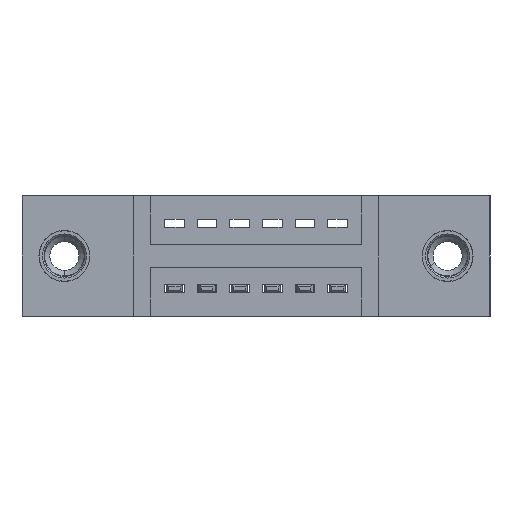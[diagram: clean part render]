
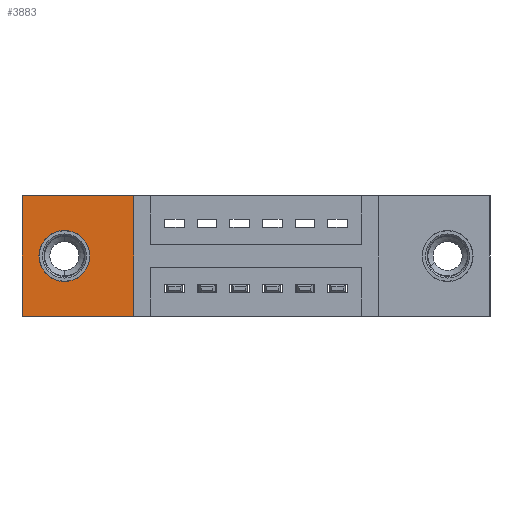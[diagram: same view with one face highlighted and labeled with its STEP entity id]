
A CAD part, front view. The second image highlights one B-rep face of the part: STEP entity #3883.
In plain terms, the highlighted planar face has unit normal (0, -1, 0).
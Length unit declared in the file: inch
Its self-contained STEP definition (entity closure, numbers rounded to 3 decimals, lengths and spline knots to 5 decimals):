
#91 = LINE ( 'NONE', #8628, #228 ) ;
#122 = DIRECTION ( 'NONE',  ( 0., -1., 0. ) ) ;
#217 = DIRECTION ( 'NONE',  ( 0., 0., -1. ) ) ;
#228 = VECTOR ( 'NONE', #3759, 39.37008 ) ;
#829 = ORIENTED_EDGE ( 'NONE', *, *, #8064, .T. ) ;
#845 = DIRECTION ( 'NONE',  ( 0., 0., -1. ) ) ;
#876 = EDGE_CURVE ( 'NONE', #2872, #4630, #8509, .T. ) ;
#2139 = ORIENTED_EDGE ( 'NONE', *, *, #2926, .T. ) ;
#2263 = FACE_BOUND ( 'NONE', #3488, .T. ) ;
#2465 = AXIS2_PLACEMENT_3D ( 'NONE', #4232, #8338, #217 ) ;
#2575 = PLANE ( 'NONE',  #2465 ) ;
#2872 = VERTEX_POINT ( 'NONE', #9754 ) ;
#2926 = EDGE_CURVE ( 'NONE', #3399, #8544, #91, .T. ) ;
#3018 = CARTESIAN_POINT ( 'NONE',  ( 0.13, 0.17, -0.185 ) ) ;
#3065 = EDGE_CURVE ( 'NONE', #5907, #3399, #10058, .T. ) ;
#3149 = ORIENTED_EDGE ( 'NONE', *, *, #876, .F. ) ;
#3399 = VERTEX_POINT ( 'NONE', #9287 ) ;
#3439 = DIRECTION ( 'NONE',  ( -1., 0., 0. ) ) ;
#3488 = EDGE_LOOP ( 'NONE', ( #5017, #3149 ) ) ;
#3630 = DIRECTION ( 'NONE',  ( 1., 0., 0. ) ) ;
#3645 = CIRCLE ( 'NONE', #3818, 0.078 ) ;
#3669 = EDGE_LOOP ( 'NONE', ( #5337, #8537, #2139, #829 ) ) ;
#3759 = DIRECTION ( 'NONE',  ( 0., 0., 1. ) ) ;
#3801 = CARTESIAN_POINT ( 'NONE',  ( 0., 0.17, 0. ) ) ;
#3818 = AXIS2_PLACEMENT_3D ( 'NONE', #3018, #7141, #4140 ) ;
#3883 = ADVANCED_FACE ( 'NONE', ( #2263, #5244 ), #2575, .T. ) ;
#3909 = DIRECTION ( 'NONE',  ( 0., 0., -1. ) ) ;
#4140 = DIRECTION ( 'NONE',  ( 0., 0., -1. ) ) ;
#4232 = CARTESIAN_POINT ( 'NONE',  ( 0., 0.17, -0.37 ) ) ;
#4376 = AXIS2_PLACEMENT_3D ( 'NONE', #5072, #122, #845 ) ;
#4400 = CARTESIAN_POINT ( 'NONE',  ( 0., 0.17, -0.37 ) ) ;
#4551 = CARTESIAN_POINT ( 'NONE',  ( 0.13, 0.17, -0.107 ) ) ;
#4630 = VERTEX_POINT ( 'NONE', #4551 ) ;
#4685 = LINE ( 'NONE', #5545, #5567 ) ;
#5017 = ORIENTED_EDGE ( 'NONE', *, *, #8403, .F. ) ;
#5072 = CARTESIAN_POINT ( 'NONE',  ( 0.13, 0.17, -0.185 ) ) ;
#5175 = LINE ( 'NONE', #8282, #7061 ) ;
#5244 = FACE_OUTER_BOUND ( 'NONE', #3669, .T. ) ;
#5337 = ORIENTED_EDGE ( 'NONE', *, *, #5396, .T. ) ;
#5396 = EDGE_CURVE ( 'NONE', #7038, #5907, #4685, .T. ) ;
#5545 = CARTESIAN_POINT ( 'NONE',  ( 0., 0.17, 0. ) ) ;
#5567 = VECTOR ( 'NONE', #3909, 39.37008 ) ;
#5907 = VERTEX_POINT ( 'NONE', #7982 ) ;
#7038 = VERTEX_POINT ( 'NONE', #3801 ) ;
#7061 = VECTOR ( 'NONE', #3439, 39.37008 ) ;
#7133 = VECTOR ( 'NONE', #3630, 39.37008 ) ;
#7141 = DIRECTION ( 'NONE',  ( 0., -1., 0. ) ) ;
#7982 = CARTESIAN_POINT ( 'NONE',  ( 0., 0.17, -0.37 ) ) ;
#8064 = EDGE_CURVE ( 'NONE', #8544, #7038, #5175, .T. ) ;
#8282 = CARTESIAN_POINT ( 'NONE',  ( 0., 0.17, 0. ) ) ;
#8338 = DIRECTION ( 'NONE',  ( 0., -1., 0. ) ) ;
#8403 = EDGE_CURVE ( 'NONE', #4630, #2872, #3645, .T. ) ;
#8509 = CIRCLE ( 'NONE', #4376, 0.078 ) ;
#8537 = ORIENTED_EDGE ( 'NONE', *, *, #3065, .T. ) ;
#8544 = VERTEX_POINT ( 'NONE', #9099 ) ;
#8628 = CARTESIAN_POINT ( 'NONE',  ( 0.3425, 0.17, 0. ) ) ;
#9099 = CARTESIAN_POINT ( 'NONE',  ( 0.3425, 0.17, 0. ) ) ;
#9287 = CARTESIAN_POINT ( 'NONE',  ( 0.3425, 0.17, -0.37 ) ) ;
#9754 = CARTESIAN_POINT ( 'NONE',  ( 0.13, 0.17, -0.263 ) ) ;
#10058 = LINE ( 'NONE', #4400, #7133 ) ;
